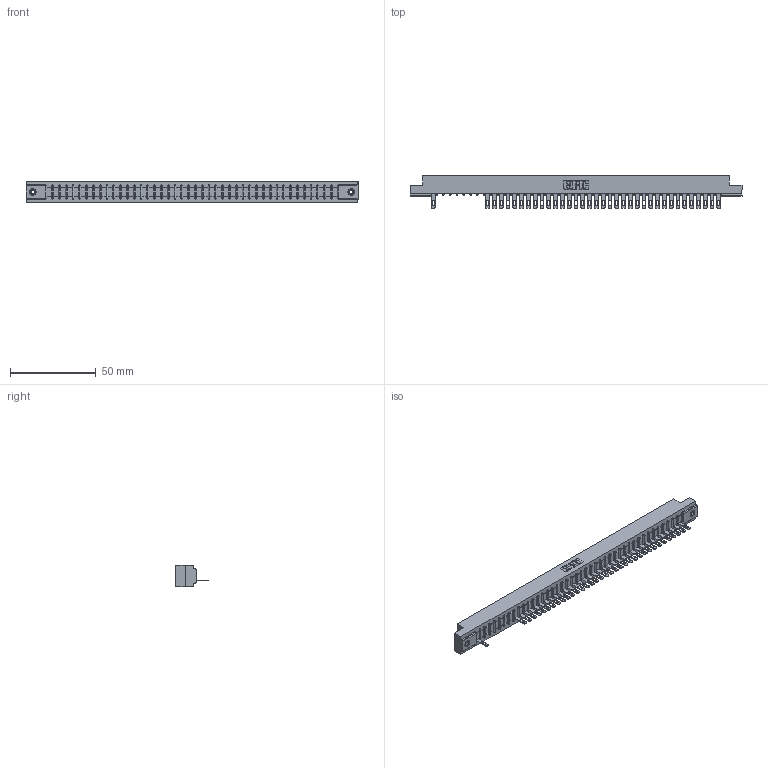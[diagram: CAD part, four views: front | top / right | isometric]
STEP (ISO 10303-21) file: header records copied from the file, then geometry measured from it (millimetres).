
FILE_DESCRIPTION (( 'STEP AP203' ), '1' );
FILE_NAME ('307-043-505-108.STEP', '2018-08-05T18:50:41', ( '' ), ( '' ), 'SwSTEP 2.0', 'SolidWorks 2016', '' );
FILE_SCHEMA (( 'CONFIG_CONTROL_DESIGN' ));
Length unit declared in the file: inch
Products named in the file (4): 307-043-505-108; 307 Part_.156 Dia Mounting Holes; 307-290-001_505; 345-250-001_345-250-003-102
Assembly tree (39 placements, depth 2):
  307-043-505-108
    307 Part_.156 Dia Mounting Holes
    307-290-001_505  x36
    345-250-001_345-250-003-102  x2
Bounding box: 193.4 x 19.18 x 12.7 mm (x, y, z)
Volume: 20023.3 mm3; surface area: 20873.9 mm2
Topology: 39 solids, 39 shells, 2378 faces, 6739 edges, 4318 vertices
Faces by surface type: plane 1482, cylinder 792, sphere 88, cone 12, torus 4
Entity records: 37675 total; most frequent: CARTESIAN_POINT 6356, ORIENTED_EDGE 6342, DIRECTION 6185, EDGE_CURVE 3171, VECTOR 2431, LINE 2431, VERTEX_POINT 2048, AXIS2_PLACEMENT_3D 1877
